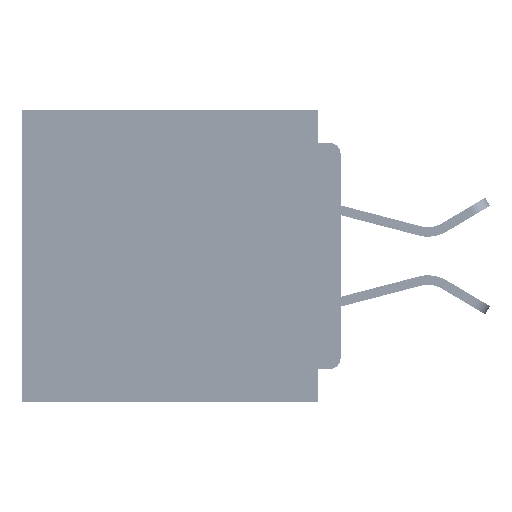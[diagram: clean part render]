
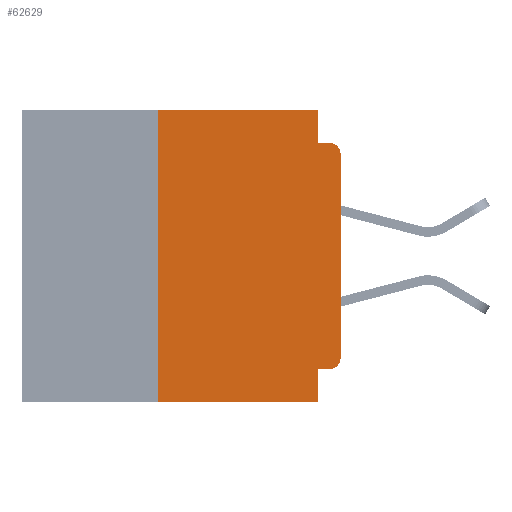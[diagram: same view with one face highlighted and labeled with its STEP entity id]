
A CAD part, left-side view. The second image highlights one B-rep face of the part: STEP entity #62629.
In plain terms, the highlighted planar face has unit normal (-1, 0, 0).
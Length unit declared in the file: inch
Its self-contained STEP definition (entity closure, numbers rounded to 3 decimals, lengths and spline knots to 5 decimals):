
#23 = CARTESIAN_POINT ( 'NONE',  ( 0., 0.25, 0. ) ) ;
#314 = CARTESIAN_POINT ( 'NONE',  ( 0., 0.015, -0.355 ) ) ;
#530 = ORIENTED_EDGE ( 'NONE', *, *, #38389, .T. ) ;
#711 = DIRECTION ( 'NONE',  ( 0., -1., 0. ) ) ;
#2978 = EDGE_CURVE ( 'NONE', #62259, #58574, #58641, .T. ) ;
#3415 = EDGE_CURVE ( 'NONE', #3558, #36440, #46261, .T. ) ;
#3558 = VERTEX_POINT ( 'NONE', #28792 ) ;
#3924 = DIRECTION ( 'NONE',  ( 0., 0., -1. ) ) ;
#3986 = DIRECTION ( 'NONE',  ( -1., 0., 0. ) ) ;
#4141 = CARTESIAN_POINT ( 'NONE',  ( 0., 0.015, -0.34 ) ) ;
#4313 = VECTOR ( 'NONE', #711, 39.37008 ) ;
#5108 = EDGE_LOOP ( 'NONE', ( #530, #47590, #51600, #49437, #48504, #27235, #23133, #10380, #41950, #61690 ) ) ;
#6903 = FACE_OUTER_BOUND ( 'NONE', #5108, .T. ) ;
#7616 = LINE ( 'NONE', #34586, #32403 ) ;
#7844 = CARTESIAN_POINT ( 'NONE',  ( 0., 0.015, -0.06 ) ) ;
#10380 = ORIENTED_EDGE ( 'NONE', *, *, #50718, .F. ) ;
#11713 = EDGE_CURVE ( 'NONE', #22473, #45695, #53918, .T. ) ;
#11970 = VECTOR ( 'NONE', #17995, 39.37008 ) ;
#12210 = CARTESIAN_POINT ( 'NONE',  ( 0., 0., -0.045 ) ) ;
#12812 = DIRECTION ( 'NONE',  ( 0., 0., -1. ) ) ;
#13046 = DIRECTION ( 'NONE',  ( 0., 0., 1. ) ) ;
#14642 = VECTOR ( 'NONE', #51823, 39.37008 ) ;
#15197 = CARTESIAN_POINT ( 'NONE',  ( 0., 0.25, -0.4 ) ) ;
#17995 = DIRECTION ( 'NONE',  ( 0., 0., -1. ) ) ;
#18236 = DIRECTION ( 'NONE',  ( 1., 0., 0. ) ) ;
#18393 = DIRECTION ( 'NONE',  ( 0., -1., 0. ) ) ;
#18687 = CARTESIAN_POINT ( 'NONE',  ( 0., 0.031, -0.355 ) ) ;
#18774 = VECTOR ( 'NONE', #53341, 39.37008 ) ;
#19117 = LINE ( 'NONE', #57840, #29196 ) ;
#19336 = VERTEX_POINT ( 'NONE', #18687 ) ;
#20411 = CARTESIAN_POINT ( 'NONE',  ( 0., 0.437, 0. ) ) ;
#20789 = LINE ( 'NONE', #22948, #45551 ) ;
#21809 = EDGE_CURVE ( 'NONE', #62259, #19336, #7616, .T. ) ;
#22473 = VERTEX_POINT ( 'NONE', #23 ) ;
#22948 = CARTESIAN_POINT ( 'NONE',  ( 0., 0., 0. ) ) ;
#23070 = CARTESIAN_POINT ( 'NONE',  ( 0., 0.25, -0.4 ) ) ;
#23133 = ORIENTED_EDGE ( 'NONE', *, *, #48355, .T. ) ;
#23434 = CARTESIAN_POINT ( 'NONE',  ( 0., 0.031, 0. ) ) ;
#23817 = LINE ( 'NONE', #15197, #38589 ) ;
#24179 = CARTESIAN_POINT ( 'NONE',  ( 0., 0.015, -0.045 ) ) ;
#24572 = AXIS2_PLACEMENT_3D ( 'NONE', #62656, #18236, #52886 ) ;
#27235 = ORIENTED_EDGE ( 'NONE', *, *, #42444, .F. ) ;
#28792 = CARTESIAN_POINT ( 'NONE',  ( 0., 0., -0.06 ) ) ;
#29196 = VECTOR ( 'NONE', #18393, 39.37008 ) ;
#29575 = DIRECTION ( 'NONE',  ( 0., 1., 0. ) ) ;
#30413 = VERTEX_POINT ( 'NONE', #23070 ) ;
#31837 = CARTESIAN_POINT ( 'NONE',  ( 0., 0., -0.34 ) ) ;
#31999 = LINE ( 'NONE', #23434, #18774 ) ;
#32403 = VECTOR ( 'NONE', #29575, 39.37008 ) ;
#32934 = CARTESIAN_POINT ( 'NONE',  ( 0., 0.031, -0.4 ) ) ;
#32980 = PLANE ( 'NONE',  #24572 ) ;
#34586 = CARTESIAN_POINT ( 'NONE',  ( 0., 0., -0.355 ) ) ;
#36440 = VERTEX_POINT ( 'NONE', #24179 ) ;
#38389 = EDGE_CURVE ( 'NONE', #58574, #3558, #20789, .T. ) ;
#38589 = VECTOR ( 'NONE', #54840, 39.37008 ) ;
#39469 = CARTESIAN_POINT ( 'NONE',  ( 0., 0.031, 0. ) ) ;
#41950 = ORIENTED_EDGE ( 'NONE', *, *, #21809, .F. ) ;
#42444 = EDGE_CURVE ( 'NONE', #30413, #22473, #23817, .T. ) ;
#42472 = DIRECTION ( 'NONE',  ( -1., 0., 0. ) ) ;
#42682 = CARTESIAN_POINT ( 'NONE',  ( 0., 0.031, -0.4 ) ) ;
#43266 = AXIS2_PLACEMENT_3D ( 'NONE', #4141, #3986, #3924 ) ;
#44307 = VERTEX_POINT ( 'NONE', #32934 ) ;
#45532 = EDGE_CURVE ( 'NONE', #45695, #59095, #31999, .T. ) ;
#45551 = VECTOR ( 'NONE', #13046, 39.37008 ) ;
#45695 = VERTEX_POINT ( 'NONE', #39469 ) ;
#46261 = CIRCLE ( 'NONE', #52034, 0.015 ) ;
#47590 = ORIENTED_EDGE ( 'NONE', *, *, #3415, .T. ) ;
#48355 = EDGE_CURVE ( 'NONE', #30413, #44307, #19117, .T. ) ;
#48504 = ORIENTED_EDGE ( 'NONE', *, *, #11713, .F. ) ;
#49437 = ORIENTED_EDGE ( 'NONE', *, *, #45532, .F. ) ;
#49898 = LINE ( 'NONE', #42682, #11970 ) ;
#50718 = EDGE_CURVE ( 'NONE', #19336, #44307, #49898, .T. ) ;
#51600 = ORIENTED_EDGE ( 'NONE', *, *, #62470, .F. ) ;
#51823 = DIRECTION ( 'NONE',  ( 0., -1., 0. ) ) ;
#52034 = AXIS2_PLACEMENT_3D ( 'NONE', #7844, #42472, #12812 ) ;
#52600 = LINE ( 'NONE', #12210, #14642 ) ;
#52886 = DIRECTION ( 'NONE',  ( 0., 0., -1. ) ) ;
#53341 = DIRECTION ( 'NONE',  ( 0., 0., -1. ) ) ;
#53918 = LINE ( 'NONE', #20411, #4313 ) ;
#54840 = DIRECTION ( 'NONE',  ( 0., 0., 1. ) ) ;
#57840 = CARTESIAN_POINT ( 'NONE',  ( 0., 0.437, -0.4 ) ) ;
#58574 = VERTEX_POINT ( 'NONE', #31837 ) ;
#58641 = CIRCLE ( 'NONE', #43266, 0.015 ) ;
#59095 = VERTEX_POINT ( 'NONE', #60142 ) ;
#60142 = CARTESIAN_POINT ( 'NONE',  ( 0., 0.031, -0.045 ) ) ;
#61690 = ORIENTED_EDGE ( 'NONE', *, *, #2978, .T. ) ;
#62259 = VERTEX_POINT ( 'NONE', #314 ) ;
#62470 = EDGE_CURVE ( 'NONE', #59095, #36440, #52600, .T. ) ;
#62629 = ADVANCED_FACE ( 'NONE', ( #6903 ), #32980, .F. ) ;
#62656 = CARTESIAN_POINT ( 'NONE',  ( 0., 0.437, 0. ) ) ;
